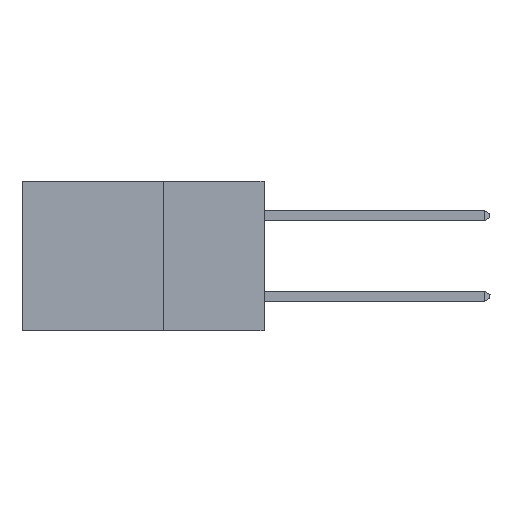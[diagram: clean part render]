
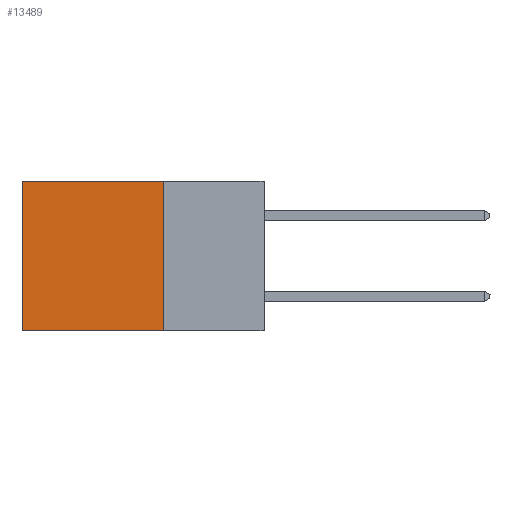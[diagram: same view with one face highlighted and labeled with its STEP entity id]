
A CAD part, left-side view. The second image highlights one B-rep face of the part: STEP entity #13489.
In plain terms, the highlighted planar face has unit normal (-1, 0, 0).
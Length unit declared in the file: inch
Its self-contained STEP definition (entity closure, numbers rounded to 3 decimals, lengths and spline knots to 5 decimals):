
#590 = LINE ( 'NONE', #3715, #6972 ) ;
#917 = LINE ( 'NONE', #1077, #10967 ) ;
#1077 = CARTESIAN_POINT ( 'NONE',  ( 0.298, 0.25, 0. ) ) ;
#2801 = VERTEX_POINT ( 'NONE', #4301 ) ;
#3321 = DIRECTION ( 'NONE',  ( 0., 1., 0. ) ) ;
#3715 = CARTESIAN_POINT ( 'NONE',  ( 0.298, 0.25, -0.37 ) ) ;
#4060 = VERTEX_POINT ( 'NONE', #6451 ) ;
#4301 = CARTESIAN_POINT ( 'NONE',  ( 0.298, 0.6, -0.37 ) ) ;
#4400 = DIRECTION ( 'NONE',  ( 1., 0., 0. ) ) ;
#4442 = FACE_OUTER_BOUND ( 'NONE', #13717, .T. ) ;
#4761 = VECTOR ( 'NONE', #5939, 39.37008 ) ;
#5353 = EDGE_CURVE ( 'NONE', #11361, #2801, #590, .T. ) ;
#5939 = DIRECTION ( 'NONE',  ( 0., 0., -1. ) ) ;
#6212 = EDGE_CURVE ( 'NONE', #4060, #10428, #917, .T. ) ;
#6451 = CARTESIAN_POINT ( 'NONE',  ( 0.298, 0.25, 0. ) ) ;
#6888 = ORIENTED_EDGE ( 'NONE', *, *, #6212, .T. ) ;
#6972 = VECTOR ( 'NONE', #10869, 39.37008 ) ;
#6986 = EDGE_CURVE ( 'NONE', #4060, #11361, #7876, .T. ) ;
#7626 = ORIENTED_EDGE ( 'NONE', *, *, #5353, .F. ) ;
#7876 = LINE ( 'NONE', #12970, #4761 ) ;
#7927 = DIRECTION ( 'NONE',  ( 0., 0., -1. ) ) ;
#9186 = PLANE ( 'NONE',  #9550 ) ;
#9339 = DIRECTION ( 'NONE',  ( 0., 0., -1. ) ) ;
#9383 = CARTESIAN_POINT ( 'NONE',  ( 0.298, 0.6, 0. ) ) ;
#9550 = AXIS2_PLACEMENT_3D ( 'NONE', #13820, #4400, #7927 ) ;
#10428 = VERTEX_POINT ( 'NONE', #13989 ) ;
#10543 = CARTESIAN_POINT ( 'NONE',  ( 0.298, 0.25, -0.37 ) ) ;
#10869 = DIRECTION ( 'NONE',  ( 0., 1., 0. ) ) ;
#10967 = VECTOR ( 'NONE', #3321, 39.37008 ) ;
#11158 = LINE ( 'NONE', #9383, #11682 ) ;
#11361 = VERTEX_POINT ( 'NONE', #10543 ) ;
#11682 = VECTOR ( 'NONE', #9339, 39.37008 ) ;
#12292 = ORIENTED_EDGE ( 'NONE', *, *, #6986, .F. ) ;
#12970 = CARTESIAN_POINT ( 'NONE',  ( 0.298, 0.25, 0. ) ) ;
#13080 = ORIENTED_EDGE ( 'NONE', *, *, #14649, .T. ) ;
#13489 = ADVANCED_FACE ( 'NONE', ( #4442 ), #9186, .F. ) ;
#13717 = EDGE_LOOP ( 'NONE', ( #13080, #7626, #12292, #6888 ) ) ;
#13820 = CARTESIAN_POINT ( 'NONE',  ( 0.298, 0.25, 0. ) ) ;
#13989 = CARTESIAN_POINT ( 'NONE',  ( 0.298, 0.6, 0. ) ) ;
#14649 = EDGE_CURVE ( 'NONE', #10428, #2801, #11158, .T. ) ;
